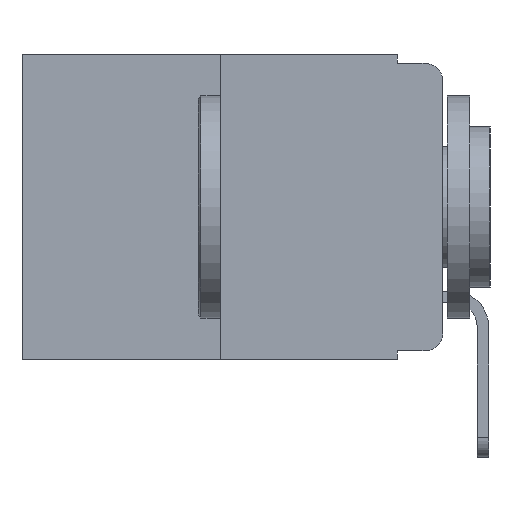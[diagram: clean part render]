
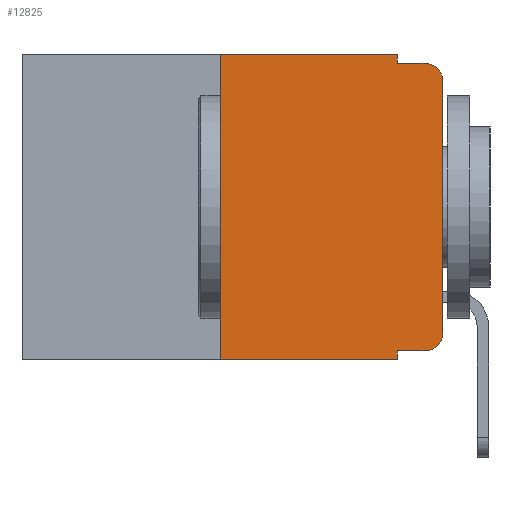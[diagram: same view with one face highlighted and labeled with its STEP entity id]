
A CAD part, left-side view. The second image highlights one B-rep face of the part: STEP entity #12825.
In plain terms, the highlighted planar face has unit normal (-1, 0, 0).
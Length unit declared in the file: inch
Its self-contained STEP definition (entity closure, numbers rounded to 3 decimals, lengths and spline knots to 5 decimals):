
#198 = EDGE_LOOP ( 'NONE', ( #4798, #10261, #5430, #3063, #6043, #8505, #8813, #4330, #5586, #11017 ) ) ;
#438 = FACE_OUTER_BOUND ( 'NONE', #198, .T. ) ;
#448 = CARTESIAN_POINT ( 'NONE',  ( 0., 0.25, -0.343 ) ) ;
#549 = CARTESIAN_POINT ( 'NONE',  ( 0., 0.02, -0.03 ) ) ;
#662 = VECTOR ( 'NONE', #3810, 39.37008 ) ;
#1010 = VECTOR ( 'NONE', #5629, 39.37008 ) ;
#1664 = DIRECTION ( 'NONE',  ( 0., 0., -1. ) ) ;
#1679 = LINE ( 'NONE', #1913, #11575 ) ;
#1759 = VECTOR ( 'NONE', #12066, 39.37008 ) ;
#1769 = EDGE_CURVE ( 'NONE', #2072, #1924, #8504, .T. ) ;
#1912 = VERTEX_POINT ( 'NONE', #10330 ) ;
#1913 = CARTESIAN_POINT ( 'NONE',  ( 0., 0.473, -0.343 ) ) ;
#1924 = VERTEX_POINT ( 'NONE', #12625 ) ;
#2072 = VERTEX_POINT ( 'NONE', #6501 ) ;
#2297 = CARTESIAN_POINT ( 'NONE',  ( 0., 0.02, -0.01 ) ) ;
#2324 = CARTESIAN_POINT ( 'NONE',  ( 0., 0.051, -0.01 ) ) ;
#2943 = DIRECTION ( 'NONE',  ( 0., 0., 1. ) ) ;
#3063 = ORIENTED_EDGE ( 'NONE', *, *, #1769, .F. ) ;
#3135 = VERTEX_POINT ( 'NONE', #6894 ) ;
#3240 = DIRECTION ( 'NONE',  ( 0., 0., -1. ) ) ;
#3383 = VECTOR ( 'NONE', #4357, 39.37008 ) ;
#3757 = AXIS2_PLACEMENT_3D ( 'NONE', #7274, #10176, #9603 ) ;
#3772 = CARTESIAN_POINT ( 'NONE',  ( 0., 0.051, -0.333 ) ) ;
#3779 = VERTEX_POINT ( 'NONE', #2297 ) ;
#3810 = DIRECTION ( 'NONE',  ( 0., -1., 0. ) ) ;
#3870 = LINE ( 'NONE', #7857, #1010 ) ;
#3958 = VERTEX_POINT ( 'NONE', #448 ) ;
#4272 = VERTEX_POINT ( 'NONE', #5731 ) ;
#4330 = ORIENTED_EDGE ( 'NONE', *, *, #6450, .F. ) ;
#4357 = DIRECTION ( 'NONE',  ( 0., -1., 0. ) ) ;
#4451 = PLANE ( 'NONE',  #9477 ) ;
#4537 = LINE ( 'NONE', #8942, #1759 ) ;
#4556 = EDGE_CURVE ( 'NONE', #5733, #3135, #11072, .T. ) ;
#4798 = ORIENTED_EDGE ( 'NONE', *, *, #9724, .T. ) ;
#4819 = CARTESIAN_POINT ( 'NONE',  ( 0., 0.051, -0.333 ) ) ;
#4891 = EDGE_CURVE ( 'NONE', #3958, #4272, #4537, .T. ) ;
#5424 = CARTESIAN_POINT ( 'NONE',  ( 0., 0.473, 0. ) ) ;
#5430 = ORIENTED_EDGE ( 'NONE', *, *, #11227, .F. ) ;
#5467 = DIRECTION ( 'NONE',  ( 0., 0., -1. ) ) ;
#5586 = ORIENTED_EDGE ( 'NONE', *, *, #6944, .T. ) ;
#5616 = EDGE_CURVE ( 'NONE', #4272, #2072, #9174, .T. ) ;
#5629 = DIRECTION ( 'NONE',  ( 0., 0., -1. ) ) ;
#5729 = VECTOR ( 'NONE', #3240, 39.37008 ) ;
#5731 = CARTESIAN_POINT ( 'NONE',  ( 0., 0.25, 0. ) ) ;
#5733 = VERTEX_POINT ( 'NONE', #5788 ) ;
#5788 = CARTESIAN_POINT ( 'NONE',  ( 0., 0.02, -0.333 ) ) ;
#5911 = AXIS2_PLACEMENT_3D ( 'NONE', #549, #7674, #1664 ) ;
#6043 = ORIENTED_EDGE ( 'NONE', *, *, #5616, .F. ) ;
#6125 = CIRCLE ( 'NONE', #5911, 0.02 ) ;
#6262 = VECTOR ( 'NONE', #2943, 39.37008 ) ;
#6360 = LINE ( 'NONE', #2324, #3383 ) ;
#6450 = EDGE_CURVE ( 'NONE', #12499, #1912, #3870, .T. ) ;
#6501 = CARTESIAN_POINT ( 'NONE',  ( 0., 0.051, 0. ) ) ;
#6680 = VECTOR ( 'NONE', #11155, 39.37008 ) ;
#6894 = CARTESIAN_POINT ( 'NONE',  ( 0., 0., -0.313 ) ) ;
#6944 = EDGE_CURVE ( 'NONE', #12499, #5733, #11308, .T. ) ;
#7274 = CARTESIAN_POINT ( 'NONE',  ( 0., 0.02, -0.313 ) ) ;
#7674 = DIRECTION ( 'NONE',  ( -1., 0., 0. ) ) ;
#7825 = CARTESIAN_POINT ( 'NONE',  ( 0., 0., 0. ) ) ;
#7857 = CARTESIAN_POINT ( 'NONE',  ( 0., 0.051, 0. ) ) ;
#8303 = VERTEX_POINT ( 'NONE', #12384 ) ;
#8504 = LINE ( 'NONE', #11317, #5729 ) ;
#8505 = ORIENTED_EDGE ( 'NONE', *, *, #4891, .F. ) ;
#8813 = ORIENTED_EDGE ( 'NONE', *, *, #12603, .T. ) ;
#8942 = CARTESIAN_POINT ( 'NONE',  ( 0., 0.25, 0. ) ) ;
#9043 = LINE ( 'NONE', #7825, #6262 ) ;
#9174 = LINE ( 'NONE', #11067, #6680 ) ;
#9287 = EDGE_CURVE ( 'NONE', #8303, #3779, #6125, .T. ) ;
#9477 = AXIS2_PLACEMENT_3D ( 'NONE', #5424, #11232, #5467 ) ;
#9603 = DIRECTION ( 'NONE',  ( 0., 0., -1. ) ) ;
#9724 = EDGE_CURVE ( 'NONE', #3135, #8303, #9043, .T. ) ;
#10176 = DIRECTION ( 'NONE',  ( -1., 0., 0. ) ) ;
#10261 = ORIENTED_EDGE ( 'NONE', *, *, #9287, .T. ) ;
#10330 = CARTESIAN_POINT ( 'NONE',  ( 0., 0.051, -0.343 ) ) ;
#10815 = DIRECTION ( 'NONE',  ( 0., -1., 0. ) ) ;
#11017 = ORIENTED_EDGE ( 'NONE', *, *, #4556, .T. ) ;
#11067 = CARTESIAN_POINT ( 'NONE',  ( 0., 0.473, 0. ) ) ;
#11072 = CIRCLE ( 'NONE', #3757, 0.02 ) ;
#11155 = DIRECTION ( 'NONE',  ( 0., -1., 0. ) ) ;
#11227 = EDGE_CURVE ( 'NONE', #1924, #3779, #6360, .T. ) ;
#11232 = DIRECTION ( 'NONE',  ( 1., 0., 0. ) ) ;
#11308 = LINE ( 'NONE', #3772, #662 ) ;
#11317 = CARTESIAN_POINT ( 'NONE',  ( 0., 0.051, 0. ) ) ;
#11575 = VECTOR ( 'NONE', #10815, 39.37008 ) ;
#12066 = DIRECTION ( 'NONE',  ( 0., 0., 1. ) ) ;
#12384 = CARTESIAN_POINT ( 'NONE',  ( 0., 0., -0.03 ) ) ;
#12499 = VERTEX_POINT ( 'NONE', #4819 ) ;
#12603 = EDGE_CURVE ( 'NONE', #3958, #1912, #1679, .T. ) ;
#12625 = CARTESIAN_POINT ( 'NONE',  ( 0., 0.051, -0.01 ) ) ;
#12825 = ADVANCED_FACE ( 'NONE', ( #438 ), #4451, .F. ) ;
